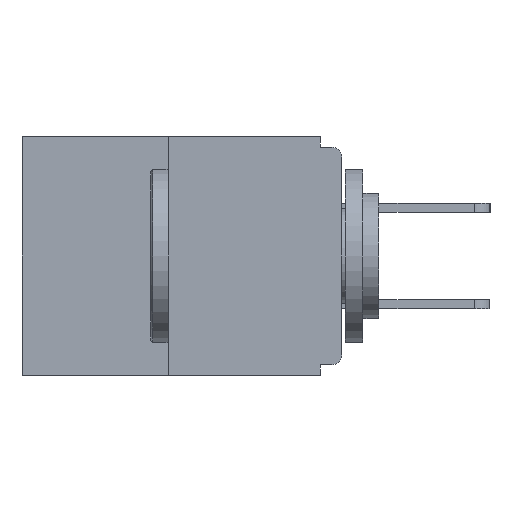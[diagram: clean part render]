
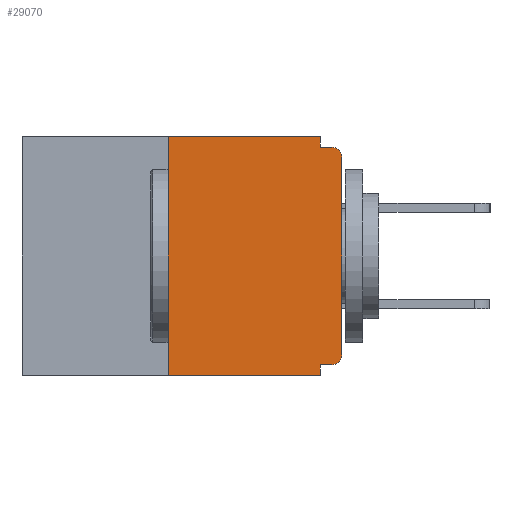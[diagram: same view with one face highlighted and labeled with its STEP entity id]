
A CAD part, left-side view. The second image highlights one B-rep face of the part: STEP entity #29070.
In plain terms, the highlighted planar face has unit normal (-1, 0, 0).
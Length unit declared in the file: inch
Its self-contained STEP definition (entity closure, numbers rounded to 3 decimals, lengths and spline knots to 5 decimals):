
#182 = DIRECTION ( 'NONE',  ( 0., 1., 0. ) ) ;
#1664 = VERTEX_POINT ( 'NONE', #24062 ) ;
#1790 = DIRECTION ( 'NONE',  ( 0., 0., 1. ) ) ;
#1835 = DIRECTION ( 'NONE',  ( 0., 0., 1. ) ) ;
#1926 = CARTESIAN_POINT ( 'NONE',  ( 0., 0., 0. ) ) ;
#2320 = VECTOR ( 'NONE', #20352, 39.37008 ) ;
#2525 = CARTESIAN_POINT ( 'NONE',  ( 0., 0.46, 0. ) ) ;
#3272 = ORIENTED_EDGE ( 'NONE', *, *, #15272, .F. ) ;
#3388 = CARTESIAN_POINT ( 'NONE',  ( 0., 0.031, -0.015 ) ) ;
#3566 = LINE ( 'NONE', #13559, #18996 ) ;
#3702 = VERTEX_POINT ( 'NONE', #7518 ) ;
#3829 = CARTESIAN_POINT ( 'NONE',  ( 0., 0.015, -0.015 ) ) ;
#4895 = DIRECTION ( 'NONE',  ( 1., 0., 0. ) ) ;
#5033 = ORIENTED_EDGE ( 'NONE', *, *, #23197, .T. ) ;
#5250 = CARTESIAN_POINT ( 'NONE',  ( 0., 0.25, 0. ) ) ;
#5317 = DIRECTION ( 'NONE',  ( 0., 0., -1. ) ) ;
#5465 = EDGE_CURVE ( 'NONE', #23473, #28924, #24489, .T. ) ;
#5588 = ORIENTED_EDGE ( 'NONE', *, *, #13293, .T. ) ;
#5777 = VECTOR ( 'NONE', #18487, 39.37008 ) ;
#7518 = CARTESIAN_POINT ( 'NONE',  ( 0., 0., -0.03 ) ) ;
#8332 = ORIENTED_EDGE ( 'NONE', *, *, #13150, .F. ) ;
#8780 = CARTESIAN_POINT ( 'NONE',  ( 0., 0.25, 0. ) ) ;
#8952 = ORIENTED_EDGE ( 'NONE', *, *, #14538, .F. ) ;
#9372 = CIRCLE ( 'NONE', #27015, 0.015 ) ;
#9638 = LINE ( 'NONE', #10641, #23631 ) ;
#9833 = CARTESIAN_POINT ( 'NONE',  ( 0., 0.031, -0.343 ) ) ;
#9893 = CARTESIAN_POINT ( 'NONE',  ( 0., 0., -0.313 ) ) ;
#9980 = CARTESIAN_POINT ( 'NONE',  ( 0., 0.015, -0.328 ) ) ;
#10027 = CARTESIAN_POINT ( 'NONE',  ( 0., 0., -0.015 ) ) ;
#10332 = AXIS2_PLACEMENT_3D ( 'NONE', #22542, #13387, #27115 ) ;
#10641 = CARTESIAN_POINT ( 'NONE',  ( 0., 0.46, -0.343 ) ) ;
#11141 = EDGE_CURVE ( 'NONE', #23187, #14961, #14641, .T. ) ;
#11240 = VECTOR ( 'NONE', #5317, 39.37008 ) ;
#11725 = LINE ( 'NONE', #24951, #5777 ) ;
#11988 = CARTESIAN_POINT ( 'NONE',  ( 0., 0.031, -0.343 ) ) ;
#12286 = DIRECTION ( 'NONE',  ( 0., -1., 0. ) ) ;
#12650 = LINE ( 'NONE', #9833, #11240 ) ;
#13150 = EDGE_CURVE ( 'NONE', #1664, #23473, #11725, .T. ) ;
#13293 = EDGE_CURVE ( 'NONE', #23187, #28431, #9638, .T. ) ;
#13387 = DIRECTION ( 'NONE',  ( -1., 0., 0. ) ) ;
#13499 = CARTESIAN_POINT ( 'NONE',  ( 0., 0.015, -0.03 ) ) ;
#13559 = CARTESIAN_POINT ( 'NONE',  ( 0., 0., -0.328 ) ) ;
#13806 = PLANE ( 'NONE',  #18750 ) ;
#14538 = EDGE_CURVE ( 'NONE', #23410, #18754, #3566, .T. ) ;
#14641 = LINE ( 'NONE', #8780, #16019 ) ;
#14951 = LINE ( 'NONE', #2525, #2320 ) ;
#14961 = VERTEX_POINT ( 'NONE', #5250 ) ;
#15272 = EDGE_CURVE ( 'NONE', #18754, #28431, #12650, .T. ) ;
#16019 = VECTOR ( 'NONE', #1790, 39.37008 ) ;
#18189 = EDGE_CURVE ( 'NONE', #3702, #28924, #9372, .T. ) ;
#18191 = VECTOR ( 'NONE', #1835, 39.37008 ) ;
#18487 = DIRECTION ( 'NONE',  ( 0., 0., -1. ) ) ;
#18527 = VECTOR ( 'NONE', #12286, 39.37008 ) ;
#18692 = DIRECTION ( 'NONE',  ( -1., 0., 0. ) ) ;
#18750 = AXIS2_PLACEMENT_3D ( 'NONE', #24975, #4895, #25265 ) ;
#18754 = VERTEX_POINT ( 'NONE', #23098 ) ;
#18996 = VECTOR ( 'NONE', #182, 39.37008 ) ;
#20352 = DIRECTION ( 'NONE',  ( 0., -1., 0. ) ) ;
#20835 = EDGE_CURVE ( 'NONE', #23410, #28198, #21095, .T. ) ;
#21095 = CIRCLE ( 'NONE', #10332, 0.015 ) ;
#21290 = ORIENTED_EDGE ( 'NONE', *, *, #20835, .T. ) ;
#21744 = ORIENTED_EDGE ( 'NONE', *, *, #18189, .T. ) ;
#22542 = CARTESIAN_POINT ( 'NONE',  ( 0., 0.015, -0.313 ) ) ;
#23098 = CARTESIAN_POINT ( 'NONE',  ( 0., 0.031, -0.328 ) ) ;
#23187 = VERTEX_POINT ( 'NONE', #24375 ) ;
#23197 = EDGE_CURVE ( 'NONE', #28198, #3702, #24153, .T. ) ;
#23276 = ORIENTED_EDGE ( 'NONE', *, *, #11141, .F. ) ;
#23410 = VERTEX_POINT ( 'NONE', #9980 ) ;
#23473 = VERTEX_POINT ( 'NONE', #3388 ) ;
#23631 = VECTOR ( 'NONE', #26119, 39.37008 ) ;
#24062 = CARTESIAN_POINT ( 'NONE',  ( 0., 0.031, 0. ) ) ;
#24153 = LINE ( 'NONE', #1926, #18191 ) ;
#24375 = CARTESIAN_POINT ( 'NONE',  ( 0., 0.25, -0.343 ) ) ;
#24407 = EDGE_LOOP ( 'NONE', ( #24855, #23276, #5588, #3272, #8952, #21290, #5033, #21744, #28676, #8332 ) ) ;
#24489 = LINE ( 'NONE', #10027, #18527 ) ;
#24753 = DIRECTION ( 'NONE',  ( 0., 0., -1. ) ) ;
#24855 = ORIENTED_EDGE ( 'NONE', *, *, #26599, .F. ) ;
#24951 = CARTESIAN_POINT ( 'NONE',  ( 0., 0.031, 0. ) ) ;
#24975 = CARTESIAN_POINT ( 'NONE',  ( 0., 0.46, 0. ) ) ;
#25265 = DIRECTION ( 'NONE',  ( 0., 0., -1. ) ) ;
#26119 = DIRECTION ( 'NONE',  ( 0., -1., 0. ) ) ;
#26599 = EDGE_CURVE ( 'NONE', #14961, #1664, #14951, .T. ) ;
#26911 = FACE_OUTER_BOUND ( 'NONE', #24407, .T. ) ;
#27015 = AXIS2_PLACEMENT_3D ( 'NONE', #13499, #18692, #24753 ) ;
#27115 = DIRECTION ( 'NONE',  ( 0., 0., -1. ) ) ;
#28198 = VERTEX_POINT ( 'NONE', #9893 ) ;
#28431 = VERTEX_POINT ( 'NONE', #11988 ) ;
#28676 = ORIENTED_EDGE ( 'NONE', *, *, #5465, .F. ) ;
#28924 = VERTEX_POINT ( 'NONE', #3829 ) ;
#29070 = ADVANCED_FACE ( 'NONE', ( #26911 ), #13806, .F. ) ;
